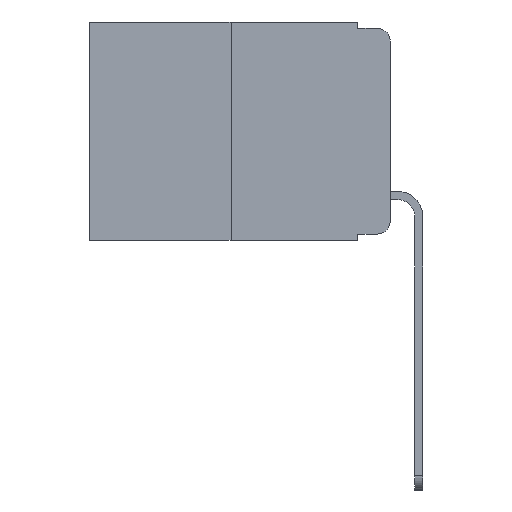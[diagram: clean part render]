
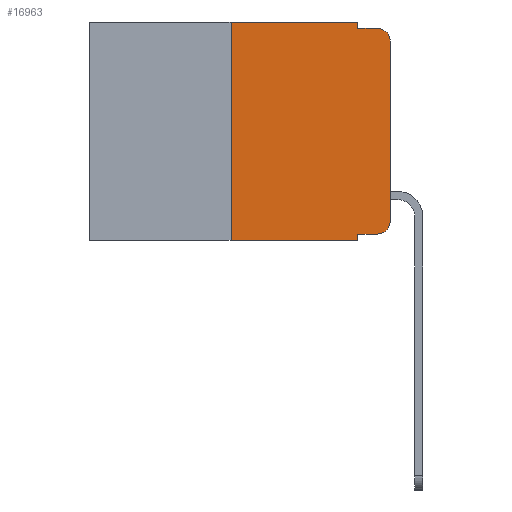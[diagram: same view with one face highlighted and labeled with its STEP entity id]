
A CAD part, left-side view. The second image highlights one B-rep face of the part: STEP entity #16963.
In plain terms, the highlighted planar face has unit normal (-1, 0, 0).
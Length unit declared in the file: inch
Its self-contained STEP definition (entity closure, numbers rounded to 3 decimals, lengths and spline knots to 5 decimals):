
#152 = AXIS2_PLACEMENT_3D ( 'NONE', #7179, #16395, #5788 ) ;
#465 = VERTEX_POINT ( 'NONE', #16230 ) ;
#502 = LINE ( 'NONE', #4092, #7722 ) ;
#1175 = VERTEX_POINT ( 'NONE', #12864 ) ;
#1339 = VERTEX_POINT ( 'NONE', #2470 ) ;
#1612 = CARTESIAN_POINT ( 'NONE',  ( 0., 0.051, 0. ) ) ;
#1637 = EDGE_CURVE ( 'NONE', #13911, #7905, #2166, .T. ) ;
#1817 = AXIS2_PLACEMENT_3D ( 'NONE', #3096, #6963, #12265 ) ;
#1897 = ORIENTED_EDGE ( 'NONE', *, *, #6047, .F. ) ;
#1927 = ORIENTED_EDGE ( 'NONE', *, *, #2324, .F. ) ;
#2038 = CARTESIAN_POINT ( 'NONE',  ( 0., 0.473, 0. ) ) ;
#2166 = LINE ( 'NONE', #4375, #8761 ) ;
#2324 = EDGE_CURVE ( 'NONE', #465, #1339, #10172, .T. ) ;
#2470 = CARTESIAN_POINT ( 'NONE',  ( 0., 0.02, -0.01 ) ) ;
#3096 = CARTESIAN_POINT ( 'NONE',  ( 0., 0.02, -0.03 ) ) ;
#3181 = VECTOR ( 'NONE', #3199, 39.37008 ) ;
#3199 = DIRECTION ( 'NONE',  ( 0., -1., 0. ) ) ;
#3261 = ORIENTED_EDGE ( 'NONE', *, *, #1637, .T. ) ;
#3423 = PLANE ( 'NONE',  #7760 ) ;
#3544 = DIRECTION ( 'NONE',  ( 1., 0., 0. ) ) ;
#3602 = LINE ( 'NONE', #4469, #3181 ) ;
#3609 = CARTESIAN_POINT ( 'NONE',  ( 0., 0.051, -0.333 ) ) ;
#4092 = CARTESIAN_POINT ( 'NONE',  ( 0., 0.25, 0. ) ) ;
#4375 = CARTESIAN_POINT ( 'NONE',  ( 0., 0.473, -0.343 ) ) ;
#4469 = CARTESIAN_POINT ( 'NONE',  ( 0., 0.051, -0.333 ) ) ;
#4584 = CARTESIAN_POINT ( 'NONE',  ( 0., 0.25, -0.343 ) ) ;
#5499 = DIRECTION ( 'NONE',  ( 0., 0., 1. ) ) ;
#5604 = ORIENTED_EDGE ( 'NONE', *, *, #9733, .T. ) ;
#5617 = CARTESIAN_POINT ( 'NONE',  ( 0., 0.02, -0.333 ) ) ;
#5788 = DIRECTION ( 'NONE',  ( 0., 0., -1. ) ) ;
#6047 = EDGE_CURVE ( 'NONE', #13911, #8149, #502, .T. ) ;
#6427 = FACE_OUTER_BOUND ( 'NONE', #15622, .T. ) ;
#6449 = EDGE_CURVE ( 'NONE', #13369, #7905, #7515, .T. ) ;
#6506 = CARTESIAN_POINT ( 'NONE',  ( 0., 0.051, 0. ) ) ;
#6631 = ORIENTED_EDGE ( 'NONE', *, *, #11411, .F. ) ;
#6963 = DIRECTION ( 'NONE',  ( -1., 0., 0. ) ) ;
#7045 = CARTESIAN_POINT ( 'NONE',  ( 0., 0.051, -0.01 ) ) ;
#7179 = CARTESIAN_POINT ( 'NONE',  ( 0., 0.02, -0.313 ) ) ;
#7515 = LINE ( 'NONE', #1612, #9976 ) ;
#7645 = CARTESIAN_POINT ( 'NONE',  ( 0., 0., 0. ) ) ;
#7722 = VECTOR ( 'NONE', #5499, 39.37008 ) ;
#7760 = AXIS2_PLACEMENT_3D ( 'NONE', #10030, #3544, #11406 ) ;
#7806 = ORIENTED_EDGE ( 'NONE', *, *, #11713, .F. ) ;
#7905 = VERTEX_POINT ( 'NONE', #16246 ) ;
#7943 = CIRCLE ( 'NONE', #1817, 0.02 ) ;
#8149 = VERTEX_POINT ( 'NONE', #8752 ) ;
#8221 = DIRECTION ( 'NONE',  ( 0., -1., 0. ) ) ;
#8752 = CARTESIAN_POINT ( 'NONE',  ( 0., 0.25, 0. ) ) ;
#8761 = VECTOR ( 'NONE', #8221, 39.37008 ) ;
#9170 = EDGE_CURVE ( 'NONE', #13430, #1175, #16813, .T. ) ;
#9257 = VECTOR ( 'NONE', #15540, 39.37008 ) ;
#9372 = DIRECTION ( 'NONE',  ( 0., 0., -1. ) ) ;
#9733 = EDGE_CURVE ( 'NONE', #9898, #13430, #12056, .T. ) ;
#9748 = ORIENTED_EDGE ( 'NONE', *, *, #10726, .T. ) ;
#9898 = VERTEX_POINT ( 'NONE', #5617 ) ;
#9929 = VERTEX_POINT ( 'NONE', #10437 ) ;
#9976 = VECTOR ( 'NONE', #9372, 39.37008 ) ;
#10030 = CARTESIAN_POINT ( 'NONE',  ( 0., 0.473, 0. ) ) ;
#10172 = LINE ( 'NONE', #7045, #16745 ) ;
#10437 = CARTESIAN_POINT ( 'NONE',  ( 0., 0.051, 0. ) ) ;
#10499 = LINE ( 'NONE', #2038, #13567 ) ;
#10672 = ORIENTED_EDGE ( 'NONE', *, *, #16820, .T. ) ;
#10726 = EDGE_CURVE ( 'NONE', #1175, #1339, #7943, .T. ) ;
#11303 = CARTESIAN_POINT ( 'NONE',  ( 0., 0., -0.313 ) ) ;
#11406 = DIRECTION ( 'NONE',  ( 0., 0., -1. ) ) ;
#11411 = EDGE_CURVE ( 'NONE', #9929, #465, #11545, .T. ) ;
#11545 = LINE ( 'NONE', #6506, #9257 ) ;
#11713 = EDGE_CURVE ( 'NONE', #8149, #9929, #10499, .T. ) ;
#12056 = CIRCLE ( 'NONE', #152, 0.02 ) ;
#12265 = DIRECTION ( 'NONE',  ( 0., 0., -1. ) ) ;
#12379 = ORIENTED_EDGE ( 'NONE', *, *, #6449, .F. ) ;
#12864 = CARTESIAN_POINT ( 'NONE',  ( 0., 0., -0.03 ) ) ;
#13306 = VECTOR ( 'NONE', #15476, 39.37008 ) ;
#13369 = VERTEX_POINT ( 'NONE', #3609 ) ;
#13430 = VERTEX_POINT ( 'NONE', #11303 ) ;
#13567 = VECTOR ( 'NONE', #15241, 39.37008 ) ;
#13911 = VERTEX_POINT ( 'NONE', #4584 ) ;
#15070 = ORIENTED_EDGE ( 'NONE', *, *, #9170, .T. ) ;
#15241 = DIRECTION ( 'NONE',  ( 0., -1., 0. ) ) ;
#15476 = DIRECTION ( 'NONE',  ( 0., 0., 1. ) ) ;
#15540 = DIRECTION ( 'NONE',  ( 0., 0., -1. ) ) ;
#15622 = EDGE_LOOP ( 'NONE', ( #15070, #9748, #1927, #6631, #7806, #1897, #3261, #12379, #10672, #5604 ) ) ;
#16194 = DIRECTION ( 'NONE',  ( 0., -1., 0. ) ) ;
#16230 = CARTESIAN_POINT ( 'NONE',  ( 0., 0.051, -0.01 ) ) ;
#16246 = CARTESIAN_POINT ( 'NONE',  ( 0., 0.051, -0.343 ) ) ;
#16395 = DIRECTION ( 'NONE',  ( -1., 0., 0. ) ) ;
#16745 = VECTOR ( 'NONE', #16194, 39.37008 ) ;
#16813 = LINE ( 'NONE', #7645, #13306 ) ;
#16820 = EDGE_CURVE ( 'NONE', #13369, #9898, #3602, .T. ) ;
#16963 = ADVANCED_FACE ( 'NONE', ( #6427 ), #3423, .F. ) ;
